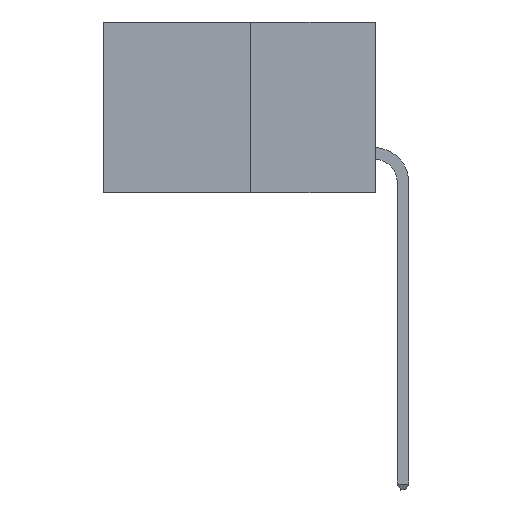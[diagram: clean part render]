
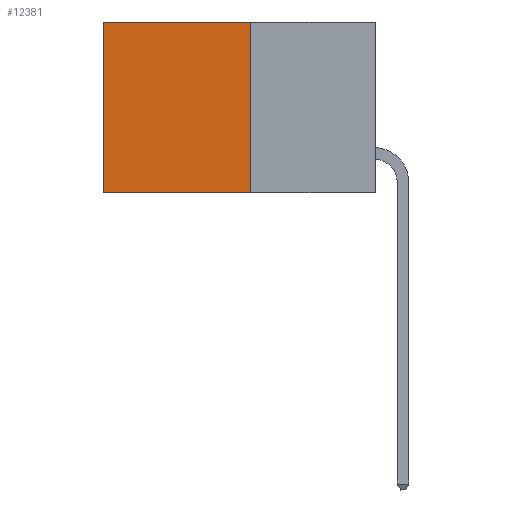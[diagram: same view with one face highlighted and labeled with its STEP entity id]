
A CAD part, left-side view. The second image highlights one B-rep face of the part: STEP entity #12381.
In plain terms, the highlighted planar face has unit normal (-1, 0, 0).
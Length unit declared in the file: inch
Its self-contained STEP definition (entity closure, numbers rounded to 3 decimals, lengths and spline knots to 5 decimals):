
#103 = DIRECTION ( 'NONE',  ( 1., 0., 0. ) ) ;
#2675 = DIRECTION ( 'NONE',  ( 0., 1., 0. ) ) ;
#3196 = LINE ( 'NONE', #17621, #16472 ) ;
#3395 = LINE ( 'NONE', #17424, #5150 ) ;
#3585 = CARTESIAN_POINT ( 'NONE',  ( 0.277, 0.27, -0.37 ) ) ;
#4163 = CARTESIAN_POINT ( 'NONE',  ( 0.277, 0.27, 0. ) ) ;
#4257 = ORIENTED_EDGE ( 'NONE', *, *, #20873, .F. ) ;
#5150 = VECTOR ( 'NONE', #19945, 39.37008 ) ;
#5305 = LINE ( 'NONE', #17402, #10381 ) ;
#5851 = FACE_OUTER_BOUND ( 'NONE', #24863, .T. ) ;
#8736 = EDGE_CURVE ( 'NONE', #26638, #21462, #26371, .T. ) ;
#9581 = EDGE_CURVE ( 'NONE', #21462, #16672, #5305, .T. ) ;
#10381 = VECTOR ( 'NONE', #19932, 39.37008 ) ;
#10744 = AXIS2_PLACEMENT_3D ( 'NONE', #29881, #103, #17593 ) ;
#10807 = ORIENTED_EDGE ( 'NONE', *, *, #11641, .F. ) ;
#11641 = EDGE_CURVE ( 'NONE', #26638, #25178, #3395, .T. ) ;
#11929 = DIRECTION ( 'NONE',  ( 0., 1., 0. ) ) ;
#12381 = ADVANCED_FACE ( 'NONE', ( #5851 ), #22515, .F. ) ;
#13958 = VECTOR ( 'NONE', #11929, 39.37008 ) ;
#16472 = VECTOR ( 'NONE', #2675, 39.37008 ) ;
#16672 = VERTEX_POINT ( 'NONE', #27635 ) ;
#17402 = CARTESIAN_POINT ( 'NONE',  ( 0.277, 0.59, -0.37 ) ) ;
#17424 = CARTESIAN_POINT ( 'NONE',  ( 0.277, 0.27, -0.37 ) ) ;
#17593 = DIRECTION ( 'NONE',  ( 0., 0., -1. ) ) ;
#17621 = CARTESIAN_POINT ( 'NONE',  ( 0.277, 0.27, -0.37 ) ) ;
#19932 = DIRECTION ( 'NONE',  ( 0., 0., -1. ) ) ;
#19945 = DIRECTION ( 'NONE',  ( 0., 0., -1. ) ) ;
#20873 = EDGE_CURVE ( 'NONE', #25178, #16672, #3196, .T. ) ;
#21462 = VERTEX_POINT ( 'NONE', #22173 ) ;
#22173 = CARTESIAN_POINT ( 'NONE',  ( 0.277, 0.59, 0. ) ) ;
#22515 = PLANE ( 'NONE',  #10744 ) ;
#24863 = EDGE_LOOP ( 'NONE', ( #30984, #4257, #10807, #29159 ) ) ;
#25178 = VERTEX_POINT ( 'NONE', #3585 ) ;
#26371 = LINE ( 'NONE', #29213, #13958 ) ;
#26638 = VERTEX_POINT ( 'NONE', #4163 ) ;
#27635 = CARTESIAN_POINT ( 'NONE',  ( 0.277, 0.59, -0.37 ) ) ;
#29159 = ORIENTED_EDGE ( 'NONE', *, *, #8736, .T. ) ;
#29213 = CARTESIAN_POINT ( 'NONE',  ( 0.277, 0.27, 0. ) ) ;
#29881 = CARTESIAN_POINT ( 'NONE',  ( 0.277, 0.27, -0.37 ) ) ;
#30984 = ORIENTED_EDGE ( 'NONE', *, *, #9581, .T. ) ;
